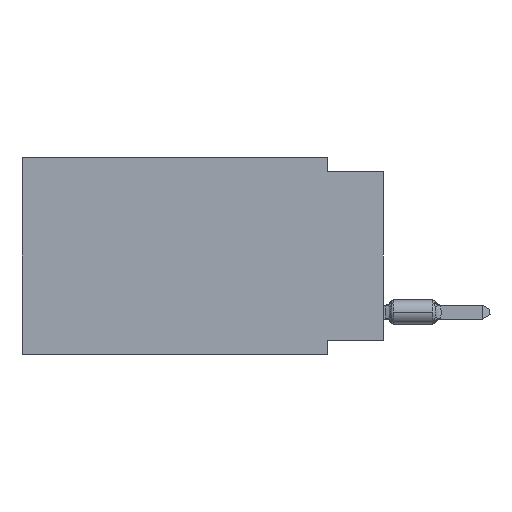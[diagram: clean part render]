
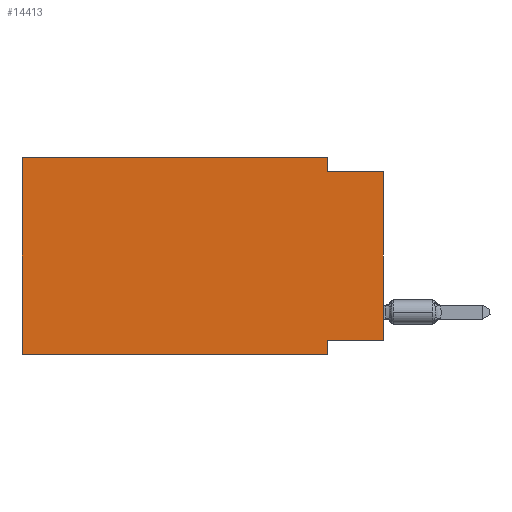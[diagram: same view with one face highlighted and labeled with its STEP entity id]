
A CAD part, left-side view. The second image highlights one B-rep face of the part: STEP entity #14413.
In plain terms, the highlighted planar face has unit normal (-1, 0, 0).
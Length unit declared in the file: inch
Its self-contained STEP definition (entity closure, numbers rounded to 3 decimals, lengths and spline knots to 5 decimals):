
#291 = CARTESIAN_POINT ( 'NONE',  ( 0., 0.645, 0. ) ) ;
#435 = LINE ( 'NONE', #627, #25987 ) ;
#627 = CARTESIAN_POINT ( 'NONE',  ( 0., 0., 0. ) ) ;
#2099 = DIRECTION ( 'NONE',  ( 0., 1., 0. ) ) ;
#2213 = ORIENTED_EDGE ( 'NONE', *, *, #13372, .F. ) ;
#3189 = EDGE_CURVE ( 'NONE', #14019, #10917, #435, .T. ) ;
#3790 = PLANE ( 'NONE',  #19309 ) ;
#4308 = VERTEX_POINT ( 'NONE', #17745 ) ;
#4803 = CARTESIAN_POINT ( 'NONE',  ( 0., 0.645, 0. ) ) ;
#7559 = CARTESIAN_POINT ( 'NONE',  ( 0., 0.1, -0.35 ) ) ;
#7748 = ORIENTED_EDGE ( 'NONE', *, *, #36192, .F. ) ;
#8049 = VECTOR ( 'NONE', #11359, 39.37008 ) ;
#8204 = EDGE_CURVE ( 'NONE', #21091, #18059, #27672, .T. ) ;
#9525 = EDGE_CURVE ( 'NONE', #13724, #32096, #20442, .T. ) ;
#9552 = DIRECTION ( 'NONE',  ( 0., 0., -1. ) ) ;
#10114 = EDGE_CURVE ( 'NONE', #21091, #13724, #19042, .T. ) ;
#10600 = CARTESIAN_POINT ( 'NONE',  ( 0., 0.1, -0.325 ) ) ;
#10823 = CARTESIAN_POINT ( 'NONE',  ( 0., 0.1, 0. ) ) ;
#10917 = VERTEX_POINT ( 'NONE', #15997 ) ;
#11359 = DIRECTION ( 'NONE',  ( 0., 0., -1. ) ) ;
#12139 = FACE_OUTER_BOUND ( 'NONE', #16119, .T. ) ;
#12333 = VECTOR ( 'NONE', #33164, 39.37008 ) ;
#13091 = EDGE_CURVE ( 'NONE', #31015, #18059, #33529, .T. ) ;
#13372 = EDGE_CURVE ( 'NONE', #14019, #31015, #32343, .T. ) ;
#13724 = VERTEX_POINT ( 'NONE', #4803 ) ;
#13747 = DIRECTION ( 'NONE',  ( 0., -1., 0. ) ) ;
#14019 = VERTEX_POINT ( 'NONE', #25749 ) ;
#14413 = ADVANCED_FACE ( 'NONE', ( #12139 ), #3790, .F. ) ;
#14900 = DIRECTION ( 'NONE',  ( 0., 0., 1. ) ) ;
#15453 = CARTESIAN_POINT ( 'NONE',  ( 0., 0., -0.325 ) ) ;
#15997 = CARTESIAN_POINT ( 'NONE',  ( 0., 0., -0.025 ) ) ;
#16119 = EDGE_LOOP ( 'NONE', ( #36118, #7748, #27867, #32110, #18156, #33191, #16303, #2213 ) ) ;
#16303 = ORIENTED_EDGE ( 'NONE', *, *, #13091, .F. ) ;
#17745 = CARTESIAN_POINT ( 'NONE',  ( 0., 0.1, -0.025 ) ) ;
#18059 = VERTEX_POINT ( 'NONE', #27368 ) ;
#18156 = ORIENTED_EDGE ( 'NONE', *, *, #10114, .F. ) ;
#18747 = CARTESIAN_POINT ( 'NONE',  ( 0., 0.1, 0. ) ) ;
#18775 = VECTOR ( 'NONE', #30565, 39.37008 ) ;
#19042 = LINE ( 'NONE', #29631, #12333 ) ;
#19309 = AXIS2_PLACEMENT_3D ( 'NONE', #291, #34965, #9552 ) ;
#19341 = LINE ( 'NONE', #10823, #8049 ) ;
#20206 = CARTESIAN_POINT ( 'NONE',  ( 0., 0., -0.025 ) ) ;
#20372 = DIRECTION ( 'NONE',  ( 0., -1., 0. ) ) ;
#20442 = LINE ( 'NONE', #22525, #23556 ) ;
#21091 = VERTEX_POINT ( 'NONE', #28474 ) ;
#22525 = CARTESIAN_POINT ( 'NONE',  ( 0., 0.645, 0. ) ) ;
#23556 = VECTOR ( 'NONE', #34546, 39.37008 ) ;
#25749 = CARTESIAN_POINT ( 'NONE',  ( 0., 0., -0.325 ) ) ;
#25987 = VECTOR ( 'NONE', #14900, 39.37008 ) ;
#27368 = CARTESIAN_POINT ( 'NONE',  ( 0., 0.1, -0.35 ) ) ;
#27672 = LINE ( 'NONE', #33252, #27818 ) ;
#27818 = VECTOR ( 'NONE', #13747, 39.37008 ) ;
#27867 = ORIENTED_EDGE ( 'NONE', *, *, #34425, .F. ) ;
#28474 = CARTESIAN_POINT ( 'NONE',  ( 0., 0.645, -0.35 ) ) ;
#29631 = CARTESIAN_POINT ( 'NONE',  ( 0., 0.645, 0. ) ) ;
#30565 = DIRECTION ( 'NONE',  ( 0., 0., -1. ) ) ;
#31015 = VERTEX_POINT ( 'NONE', #10600 ) ;
#31239 = VECTOR ( 'NONE', #20372, 39.37008 ) ;
#32096 = VERTEX_POINT ( 'NONE', #18747 ) ;
#32110 = ORIENTED_EDGE ( 'NONE', *, *, #9525, .F. ) ;
#32343 = LINE ( 'NONE', #15453, #36010 ) ;
#33164 = DIRECTION ( 'NONE',  ( 0., 0., 1. ) ) ;
#33191 = ORIENTED_EDGE ( 'NONE', *, *, #8204, .T. ) ;
#33252 = CARTESIAN_POINT ( 'NONE',  ( 0., 0.645, -0.35 ) ) ;
#33529 = LINE ( 'NONE', #7559, #18775 ) ;
#34425 = EDGE_CURVE ( 'NONE', #32096, #4308, #19341, .T. ) ;
#34546 = DIRECTION ( 'NONE',  ( 0., -1., 0. ) ) ;
#34663 = LINE ( 'NONE', #20206, #31239 ) ;
#34965 = DIRECTION ( 'NONE',  ( 1., 0., 0. ) ) ;
#36010 = VECTOR ( 'NONE', #2099, 39.37008 ) ;
#36118 = ORIENTED_EDGE ( 'NONE', *, *, #3189, .T. ) ;
#36192 = EDGE_CURVE ( 'NONE', #4308, #10917, #34663, .T. ) ;
